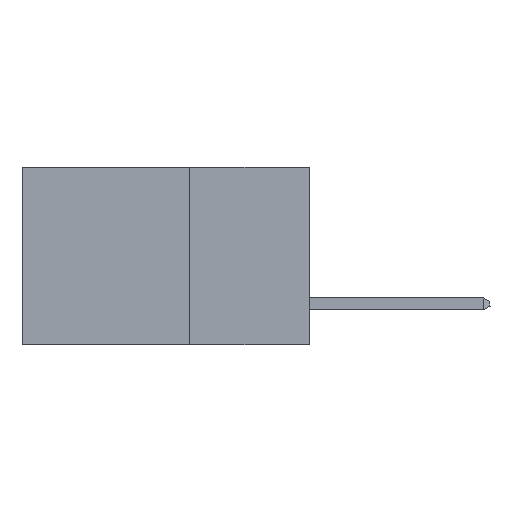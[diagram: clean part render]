
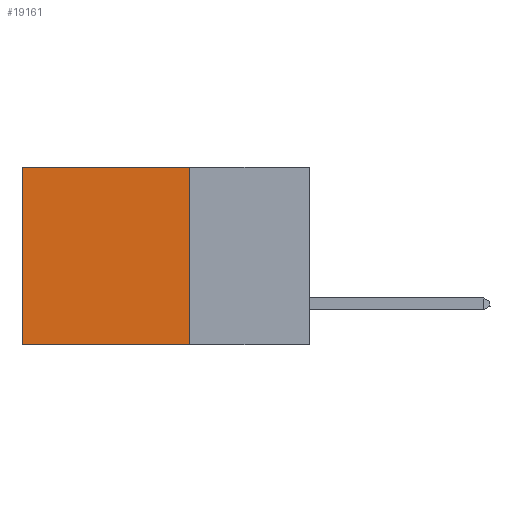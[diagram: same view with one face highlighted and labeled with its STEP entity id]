
A CAD part, left-side view. The second image highlights one B-rep face of the part: STEP entity #19161.
In plain terms, the highlighted planar face has unit normal (-1, 0, 0).
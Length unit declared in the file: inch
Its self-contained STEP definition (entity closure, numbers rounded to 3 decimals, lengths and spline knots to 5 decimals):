
#525 = VERTEX_POINT ( 'NONE', #18906 ) ;
#544 = FACE_OUTER_BOUND ( 'NONE', #12211, .T. ) ;
#945 = CARTESIAN_POINT ( 'NONE',  ( 0.2875, 0.6, 0. ) ) ;
#1436 = VERTEX_POINT ( 'NONE', #17974 ) ;
#3366 = VECTOR ( 'NONE', #3669, 39.37008 ) ;
#3669 = DIRECTION ( 'NONE',  ( 0., 1., 0. ) ) ;
#4657 = CARTESIAN_POINT ( 'NONE',  ( 0.2875, 0.6, 0. ) ) ;
#4800 = VERTEX_POINT ( 'NONE', #5847 ) ;
#5847 = CARTESIAN_POINT ( 'NONE',  ( 0.2875, 0.25, -0.37 ) ) ;
#5865 = ORIENTED_EDGE ( 'NONE', *, *, #14625, .T. ) ;
#6256 = VECTOR ( 'NONE', #21271, 39.37008 ) ;
#6399 = ORIENTED_EDGE ( 'NONE', *, *, #9859, .T. ) ;
#9859 = EDGE_CURVE ( 'NONE', #22772, #525, #15741, .T. ) ;
#11445 = ORIENTED_EDGE ( 'NONE', *, *, #14885, .F. ) ;
#11848 = VECTOR ( 'NONE', #13114, 39.37008 ) ;
#12211 = EDGE_LOOP ( 'NONE', ( #6399, #21707, #11445, #5865 ) ) ;
#12747 = CARTESIAN_POINT ( 'NONE',  ( 0.2875, 0.25, 0. ) ) ;
#12821 = CARTESIAN_POINT ( 'NONE',  ( 0.2875, 0.25, 0. ) ) ;
#13114 = DIRECTION ( 'NONE',  ( 0., 0., -1. ) ) ;
#13639 = DIRECTION ( 'NONE',  ( 0., 1., 0. ) ) ;
#14625 = EDGE_CURVE ( 'NONE', #1436, #22772, #22760, .T. ) ;
#14885 = EDGE_CURVE ( 'NONE', #1436, #4800, #25589, .T. ) ;
#15565 = EDGE_CURVE ( 'NONE', #4800, #525, #26540, .T. ) ;
#15741 = LINE ( 'NONE', #945, #11848 ) ;
#16648 = DIRECTION ( 'NONE',  ( 0., 0., -1. ) ) ;
#17974 = CARTESIAN_POINT ( 'NONE',  ( 0.2875, 0.25, 0. ) ) ;
#18881 = PLANE ( 'NONE',  #19551 ) ;
#18906 = CARTESIAN_POINT ( 'NONE',  ( 0.2875, 0.6, -0.37 ) ) ;
#19161 = ADVANCED_FACE ( 'NONE', ( #544 ), #18881, .F. ) ;
#19498 = VECTOR ( 'NONE', #13639, 39.37008 ) ;
#19551 = AXIS2_PLACEMENT_3D ( 'NONE', #12821, #20669, #16648 ) ;
#20669 = DIRECTION ( 'NONE',  ( 1., 0., 0. ) ) ;
#21271 = DIRECTION ( 'NONE',  ( 0., 0., -1. ) ) ;
#21707 = ORIENTED_EDGE ( 'NONE', *, *, #15565, .F. ) ;
#22760 = LINE ( 'NONE', #26577, #3366 ) ;
#22772 = VERTEX_POINT ( 'NONE', #4657 ) ;
#25589 = LINE ( 'NONE', #12747, #6256 ) ;
#25914 = CARTESIAN_POINT ( 'NONE',  ( 0.2875, 0.25, -0.37 ) ) ;
#26540 = LINE ( 'NONE', #25914, #19498 ) ;
#26577 = CARTESIAN_POINT ( 'NONE',  ( 0.2875, 0.25, 0. ) ) ;
